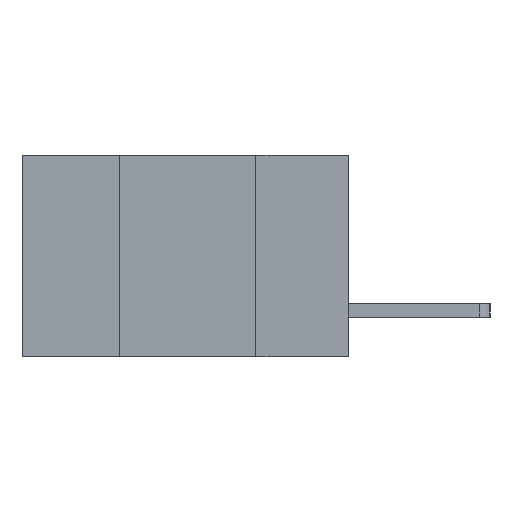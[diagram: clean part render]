
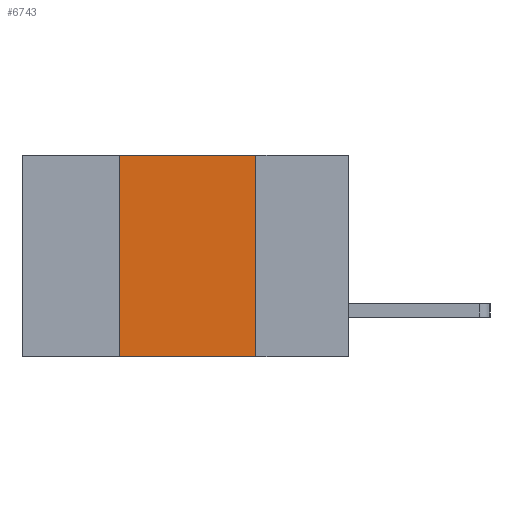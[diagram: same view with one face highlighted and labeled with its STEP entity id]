
A CAD part, left-side view. The second image highlights one B-rep face of the part: STEP entity #6743.
In plain terms, the highlighted planar face has unit normal (-1, 0, 0).
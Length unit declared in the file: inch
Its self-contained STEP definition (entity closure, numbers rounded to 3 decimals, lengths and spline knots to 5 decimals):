
#225 = CARTESIAN_POINT ( 'NONE',  ( 0., 0.6, -0.37 ) ) ;
#413 = VERTEX_POINT ( 'NONE', #9405 ) ;
#674 = CARTESIAN_POINT ( 'NONE',  ( 0., 0.6, 0. ) ) ;
#694 = VERTEX_POINT ( 'NONE', #5025 ) ;
#889 = LINE ( 'NONE', #1226, #4677 ) ;
#1226 = CARTESIAN_POINT ( 'NONE',  ( 0., 0.42, 0. ) ) ;
#1363 = VECTOR ( 'NONE', #5379, 39.37008 ) ;
#1457 = EDGE_CURVE ( 'NONE', #694, #413, #889, .T. ) ;
#1605 = VECTOR ( 'NONE', #2915, 39.37008 ) ;
#1698 = CARTESIAN_POINT ( 'NONE',  ( 0., 0.6, 0. ) ) ;
#2461 = DIRECTION ( 'NONE',  ( 0., 0., -1. ) ) ;
#2703 = EDGE_LOOP ( 'NONE', ( #5878, #4944, #9094, #4610 ) ) ;
#2915 = DIRECTION ( 'NONE',  ( 0., -1., 0. ) ) ;
#3005 = FACE_OUTER_BOUND ( 'NONE', #2703, .T. ) ;
#3113 = AXIS2_PLACEMENT_3D ( 'NONE', #1698, #6958, #2461 ) ;
#3345 = LINE ( 'NONE', #3861, #1363 ) ;
#3861 = CARTESIAN_POINT ( 'NONE',  ( 0., 0.17, 0. ) ) ;
#3937 = CARTESIAN_POINT ( 'NONE',  ( 0., 0.17, 0. ) ) ;
#4610 = ORIENTED_EDGE ( 'NONE', *, *, #5500, .T. ) ;
#4677 = VECTOR ( 'NONE', #4826, 39.37008 ) ;
#4826 = DIRECTION ( 'NONE',  ( 0., 0., 1. ) ) ;
#4899 = VERTEX_POINT ( 'NONE', #3937 ) ;
#4944 = ORIENTED_EDGE ( 'NONE', *, *, #6491, .F. ) ;
#5025 = CARTESIAN_POINT ( 'NONE',  ( 0., 0.42, -0.37 ) ) ;
#5379 = DIRECTION ( 'NONE',  ( 0., 0., -1. ) ) ;
#5500 = EDGE_CURVE ( 'NONE', #694, #7950, #8615, .T. ) ;
#5878 = ORIENTED_EDGE ( 'NONE', *, *, #7186, .F. ) ;
#6377 = VECTOR ( 'NONE', #7016, 39.37008 ) ;
#6426 = CARTESIAN_POINT ( 'NONE',  ( 0., 0.17, -0.37 ) ) ;
#6491 = EDGE_CURVE ( 'NONE', #413, #4899, #7357, .T. ) ;
#6743 = ADVANCED_FACE ( 'NONE', ( #3005 ), #9227, .F. ) ;
#6958 = DIRECTION ( 'NONE',  ( 1., 0., 0. ) ) ;
#7016 = DIRECTION ( 'NONE',  ( 0., -1., 0. ) ) ;
#7186 = EDGE_CURVE ( 'NONE', #4899, #7950, #3345, .T. ) ;
#7357 = LINE ( 'NONE', #674, #1605 ) ;
#7950 = VERTEX_POINT ( 'NONE', #6426 ) ;
#8615 = LINE ( 'NONE', #225, #6377 ) ;
#9094 = ORIENTED_EDGE ( 'NONE', *, *, #1457, .F. ) ;
#9227 = PLANE ( 'NONE',  #3113 ) ;
#9405 = CARTESIAN_POINT ( 'NONE',  ( 0., 0.42, 0. ) ) ;
